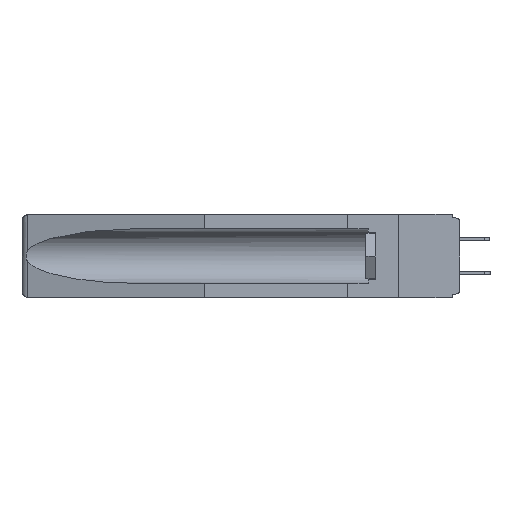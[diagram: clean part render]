
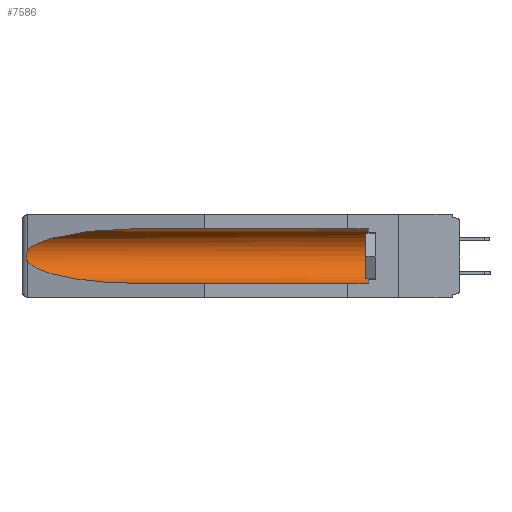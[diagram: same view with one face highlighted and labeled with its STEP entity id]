
A CAD part, left-side view. The second image highlights one B-rep face of the part: STEP entity #7586.
In plain terms, the highlighted cylindrical face has radius 2.857 mm (diameter 5.715 mm), a partial arc.
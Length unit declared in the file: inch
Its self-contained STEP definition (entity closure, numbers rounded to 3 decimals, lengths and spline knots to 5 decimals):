
#330 = VERTEX_POINT ( 'NONE', #4346 ) ;
#450 = VECTOR ( 'NONE', #5125, 39.37008 ) ;
#575 = CYLINDRICAL_SURFACE ( 'NONE', #15272, 0.1125 ) ;
#595 = AXIS2_PLACEMENT_3D ( 'NONE', #12853, #10221, #15776 ) ;
#761 = CARTESIAN_POINT ( 'NONE',  ( 0.26537, 1.52718, -0.14972 ) ) ;
#1076 = CARTESIAN_POINT ( 'NONE',  ( 0.26537, 1.52718, -0.19328 ) ) ;
#1351 = CARTESIAN_POINT ( 'NONE',  ( 0.26537, 1.52718, -0.14972 ) ) ;
#2114 = LINE ( 'NONE', #16308, #17272 ) ;
#2219 = VERTEX_POINT ( 'NONE', #6496 ) ;
#2664 = CARTESIAN_POINT ( 'NONE',  ( 0.26655, 1.53094, -0.18657 ) ) ;
#2739 = CARTESIAN_POINT ( 'NONE',  ( 0.21114, 1.30732, -0.284 ) ) ;
#2913 =( BOUNDED_CURVE ( )  B_SPLINE_CURVE ( 3, ( #10884, #3254, #14983, #761 ),
 .UNSPECIFIED., .F., .F. ) 
 B_SPLINE_CURVE_WITH_KNOTS ( ( 4, 4 ),
 ( 4.71239, 6.08839 ),
 .UNSPECIFIED. ) 
 CURVE ( )  GEOMETRIC_REPRESENTATION_ITEM ( )  RATIONAL_B_SPLINE_CURVE ( ( 1., 0.848, 0.848, 1. ) ) 
 REPRESENTATION_ITEM ( '' )  );
#2940 = CARTESIAN_POINT ( 'NONE',  ( 0.26654, 1.53092, -0.15636 ) ) ;
#3254 = CARTESIAN_POINT ( 'NONE',  ( 0.21114, 1.30732, -0.059 ) ) ;
#3901 = ORIENTED_EDGE ( 'NONE', *, *, #12395, .T. ) ;
#3971 = ORIENTED_EDGE ( 'NONE', *, *, #17374, .T. ) ;
#4184 = CARTESIAN_POINT ( 'NONE',  ( 0.2675, 1.53308, -0.17534 ) ) ;
#4346 = CARTESIAN_POINT ( 'NONE',  ( 0.155, 1.07973, -0.059 ) ) ;
#4545 = DIRECTION ( 'NONE',  ( 0., 1., 0. ) ) ;
#4702 = CARTESIAN_POINT ( 'NONE',  ( 0.26537, 1.52718, -0.14972 ) ) ;
#4917 = VERTEX_POINT ( 'NONE', #4702 ) ;
#5125 = DIRECTION ( 'NONE',  ( 0., 1., 0. ) ) ;
#5313 = ORIENTED_EDGE ( 'NONE', *, *, #17105, .F. ) ;
#5907 = CARTESIAN_POINT ( 'NONE',  ( 0.26597, 1.52961, -0.15275 ) ) ;
#6496 = CARTESIAN_POINT ( 'NONE',  ( 0.155, 1.07973, -0.284 ) ) ;
#7072 = ORIENTED_EDGE ( 'NONE', *, *, #10638, .T. ) ;
#7133 = CARTESIAN_POINT ( 'NONE',  ( 0.26537, 1.52718, -0.19328 ) ) ;
#7341 = LINE ( 'NONE', #15244, #450 ) ;
#7497 = ORIENTED_EDGE ( 'NONE', *, *, #8904, .T. ) ;
#7586 = ADVANCED_FACE ( 'NONE', ( #18025 ), #575, .F. ) ;
#8904 = EDGE_CURVE ( 'NONE', #17807, #11215, #14050, .T. ) ;
#9028 = CARTESIAN_POINT ( 'NONE',  ( 0.155, 0.126, -0.059 ) ) ;
#9120 = DIRECTION ( 'NONE',  ( 0., 0., 1. ) ) ;
#9627 = ORIENTED_EDGE ( 'NONE', *, *, #18834, .T. ) ;
#9823 = EDGE_LOOP ( 'NONE', ( #9627, #3971, #7072, #5313, #7497, #3901 ) ) ;
#10221 = DIRECTION ( 'NONE',  ( 0., -1., 0. ) ) ;
#10264 = CARTESIAN_POINT ( 'NONE',  ( 0.26597, 1.5296, -0.19026 ) ) ;
#10495 = DIRECTION ( 'NONE',  ( 0., 1., 0. ) ) ;
#10638 = EDGE_CURVE ( 'NONE', #11788, #2219, #14927, .T. ) ;
#10884 = CARTESIAN_POINT ( 'NONE',  ( 0.155, 1.07973, -0.059 ) ) ;
#11215 = VERTEX_POINT ( 'NONE', #9028 ) ;
#11552 = CARTESIAN_POINT ( 'NONE',  ( 0.25451, 1.48313, -0.24835 ) ) ;
#11788 = VERTEX_POINT ( 'NONE', #1076 ) ;
#12395 = EDGE_CURVE ( 'NONE', #11215, #330, #2114, .T. ) ;
#12853 = CARTESIAN_POINT ( 'NONE',  ( 0.155, 0.126, -0.1715 ) ) ;
#13225 = CARTESIAN_POINT ( 'NONE',  ( 0.2673, 1.5327, -0.16383 ) ) ;
#13454 = CARTESIAN_POINT ( 'NONE',  ( 0.155, -0.30754, -0.1715 ) ) ;
#14050 = CIRCLE ( 'NONE', #595, 0.1125 ) ;
#14569 = CARTESIAN_POINT ( 'NONE',  ( 0.155, 0.126, -0.284 ) ) ;
#14619 = CARTESIAN_POINT ( 'NONE',  ( 0.2675, 1.53308, -0.16763 ) ) ;
#14927 =( BOUNDED_CURVE ( )  B_SPLINE_CURVE ( 3, ( #7133, #11552, #2739, #16028 ),
 .UNSPECIFIED., .F., .F. ) 
 B_SPLINE_CURVE_WITH_KNOTS ( ( 4, 4 ),
 ( 0.1948, 1.5708 ),
 .UNSPECIFIED. ) 
 CURVE ( )  GEOMETRIC_REPRESENTATION_ITEM ( )  RATIONAL_B_SPLINE_CURVE ( ( 1., 0.848, 0.848, 1. ) ) 
 REPRESENTATION_ITEM ( '' )  );
#14983 = CARTESIAN_POINT ( 'NONE',  ( 0.25451, 1.48313, -0.09465 ) ) ;
#15244 = CARTESIAN_POINT ( 'NONE',  ( 0.155, -0.30754, -0.284 ) ) ;
#15272 = AXIS2_PLACEMENT_3D ( 'NONE', #13454, #10495, #9120 ) ;
#15776 = DIRECTION ( 'NONE',  ( 0., 0., 1. ) ) ;
#15966 = B_SPLINE_CURVE_WITH_KNOTS ( 'NONE', 3,
 ( #1351, #5907, #2940, #13225, #14619, #4184, #17634, #2664, #10264, #16151 ),
 .UNSPECIFIED., .F., .F.,
 ( 4, 2, 2, 2, 4 ),
 ( 0., 0.00029, 0.00058, 0.00087, 0.00117 ),
 .UNSPECIFIED. ) ;
#16028 = CARTESIAN_POINT ( 'NONE',  ( 0.155, 1.07973, -0.284 ) ) ;
#16151 = CARTESIAN_POINT ( 'NONE',  ( 0.26537, 1.52718, -0.19328 ) ) ;
#16308 = CARTESIAN_POINT ( 'NONE',  ( 0.155, -0.30754, -0.059 ) ) ;
#17105 = EDGE_CURVE ( 'NONE', #17807, #2219, #7341, .T. ) ;
#17272 = VECTOR ( 'NONE', #4545, 39.37008 ) ;
#17374 = EDGE_CURVE ( 'NONE', #4917, #11788, #15966, .T. ) ;
#17634 = CARTESIAN_POINT ( 'NONE',  ( 0.2673, 1.53269, -0.17917 ) ) ;
#17807 = VERTEX_POINT ( 'NONE', #14569 ) ;
#18025 = FACE_OUTER_BOUND ( 'NONE', #9823, .T. ) ;
#18834 = EDGE_CURVE ( 'NONE', #330, #4917, #2913, .T. ) ;
